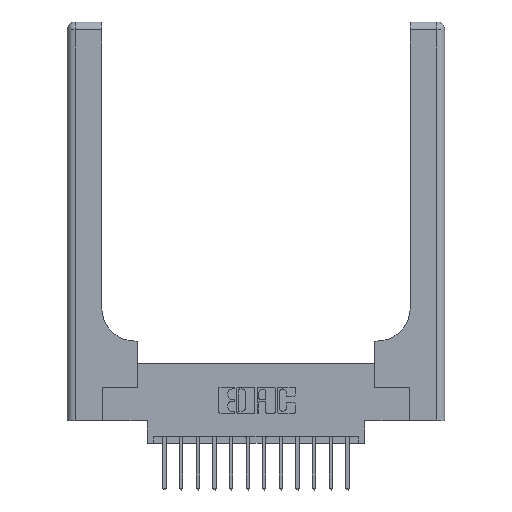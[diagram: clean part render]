
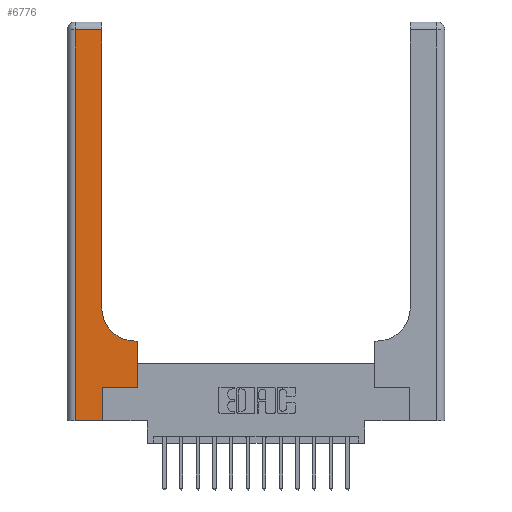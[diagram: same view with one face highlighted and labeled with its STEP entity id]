
A CAD part, top view. The second image highlights one B-rep face of the part: STEP entity #6776.
In plain terms, the highlighted planar face has unit normal (0, 0, 1).
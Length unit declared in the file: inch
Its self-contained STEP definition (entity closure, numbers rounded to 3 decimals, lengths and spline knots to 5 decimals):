
#59 = DIRECTION ( 'NONE',  ( 1., 0., 0. ) ) ;
#504 = DIRECTION ( 'NONE',  ( 0., 1., 0. ) ) ;
#699 = CARTESIAN_POINT ( 'NONE',  ( 0.265, 0.25, 0.37 ) ) ;
#1008 = PLANE ( 'NONE',  #9609 ) ;
#1213 = VERTEX_POINT ( 'NONE', #1940 ) ;
#1661 = EDGE_CURVE ( 'NONE', #13261, #1213, #16543, .T. ) ;
#1783 = LINE ( 'NONE', #15184, #11985 ) ;
#1837 = CARTESIAN_POINT ( 'NONE',  ( 0.06, 3., 0.37 ) ) ;
#1850 = FACE_OUTER_BOUND ( 'NONE', #15285, .T. ) ;
#1940 = CARTESIAN_POINT ( 'NONE',  ( 0.528, 0.25, 0.37 ) ) ;
#2339 = EDGE_CURVE ( 'NONE', #14521, #10930, #16321, .T. ) ;
#2341 = CARTESIAN_POINT ( 'NONE',  ( 0.26, 0.6, 0.37 ) ) ;
#2517 = CIRCLE ( 'NONE', #5534, 0.25 ) ;
#2592 = CARTESIAN_POINT ( 'NONE',  ( 0.528, 0.25, 0.37 ) ) ;
#2735 = CARTESIAN_POINT ( 'NONE',  ( 0.06, 2.94, 0.37 ) ) ;
#2907 = VECTOR ( 'NONE', #6356, 39.37008 ) ;
#3152 = CARTESIAN_POINT ( 'NONE',  ( 0.265, 0.25, 0.37 ) ) ;
#3167 = ORIENTED_EDGE ( 'NONE', *, *, #15888, .T. ) ;
#3273 = EDGE_CURVE ( 'NONE', #9309, #14521, #8649, .T. ) ;
#3549 = VECTOR ( 'NONE', #15789, 39.37008 ) ;
#3654 = LINE ( 'NONE', #2592, #6794 ) ;
#3976 = LINE ( 'NONE', #9172, #3549 ) ;
#4113 = VERTEX_POINT ( 'NONE', #9343 ) ;
#4684 = VERTEX_POINT ( 'NONE', #16342 ) ;
#4693 = DIRECTION ( 'NONE',  ( 1., 0., 0. ) ) ;
#5178 = ORIENTED_EDGE ( 'NONE', *, *, #13541, .T. ) ;
#5183 = VERTEX_POINT ( 'NONE', #13406 ) ;
#5332 = ORIENTED_EDGE ( 'NONE', *, *, #3273, .T. ) ;
#5534 = AXIS2_PLACEMENT_3D ( 'NONE', #15979, #8024, #59 ) ;
#5975 = ORIENTED_EDGE ( 'NONE', *, *, #2339, .T. ) ;
#6150 = EDGE_CURVE ( 'NONE', #4113, #14596, #3976, .T. ) ;
#6356 = DIRECTION ( 'NONE',  ( -1., 0., 0. ) ) ;
#6461 = LINE ( 'NONE', #2341, #2907 ) ;
#6776 = ADVANCED_FACE ( 'NONE', ( #1850 ), #1008, .F. ) ;
#6794 = VECTOR ( 'NONE', #13196, 39.37008 ) ;
#7263 = ORIENTED_EDGE ( 'NONE', *, *, #9973, .T. ) ;
#7431 = CARTESIAN_POINT ( 'NONE',  ( 0.26, 2.94, 0.37 ) ) ;
#7546 = ORIENTED_EDGE ( 'NONE', *, *, #8370, .T. ) ;
#7697 = DIRECTION ( 'NONE',  ( 0., 0., -1. ) ) ;
#7896 = DIRECTION ( 'NONE',  ( 1., 0., 0. ) ) ;
#8024 = DIRECTION ( 'NONE',  ( 0., 0., -1. ) ) ;
#8370 = EDGE_CURVE ( 'NONE', #10930, #13261, #10602, .T. ) ;
#8649 = LINE ( 'NONE', #1837, #9076 ) ;
#9076 = VECTOR ( 'NONE', #13798, 39.37008 ) ;
#9172 = CARTESIAN_POINT ( 'NONE',  ( 0.26, 3., 0.37 ) ) ;
#9239 = CARTESIAN_POINT ( 'NONE',  ( 0., 0., 0.37 ) ) ;
#9309 = VERTEX_POINT ( 'NONE', #2735 ) ;
#9343 = CARTESIAN_POINT ( 'NONE',  ( 0.26, 0.85, 0.37 ) ) ;
#9609 = AXIS2_PLACEMENT_3D ( 'NONE', #15654, #7697, #16988 ) ;
#9973 = EDGE_CURVE ( 'NONE', #14596, #9309, #1783, .T. ) ;
#10602 = LINE ( 'NONE', #16417, #13731 ) ;
#10930 = VERTEX_POINT ( 'NONE', #14872 ) ;
#11985 = VECTOR ( 'NONE', #16503, 39.37008 ) ;
#12174 = ORIENTED_EDGE ( 'NONE', *, *, #6150, .T. ) ;
#12600 = CARTESIAN_POINT ( 'NONE',  ( 0.06, 0., 0.37 ) ) ;
#12798 = VECTOR ( 'NONE', #7896, 39.37008 ) ;
#13014 = EDGE_CURVE ( 'NONE', #5183, #4113, #2517, .T. ) ;
#13028 = VECTOR ( 'NONE', #4693, 39.37008 ) ;
#13103 = ORIENTED_EDGE ( 'NONE', *, *, #1661, .T. ) ;
#13196 = DIRECTION ( 'NONE',  ( 0., 1., 0. ) ) ;
#13261 = VERTEX_POINT ( 'NONE', #3152 ) ;
#13406 = CARTESIAN_POINT ( 'NONE',  ( 0.51, 0.6, 0.37 ) ) ;
#13541 = EDGE_CURVE ( 'NONE', #4684, #5183, #6461, .T. ) ;
#13731 = VECTOR ( 'NONE', #504, 39.37008 ) ;
#13798 = DIRECTION ( 'NONE',  ( 0., -1., 0. ) ) ;
#14521 = VERTEX_POINT ( 'NONE', #12600 ) ;
#14596 = VERTEX_POINT ( 'NONE', #7431 ) ;
#14872 = CARTESIAN_POINT ( 'NONE',  ( 0.265, 0., 0.37 ) ) ;
#15184 = CARTESIAN_POINT ( 'NONE',  ( 0., 2.94, 0.37 ) ) ;
#15285 = EDGE_LOOP ( 'NONE', ( #12174, #7263, #5332, #5975, #7546, #13103, #3167, #5178, #16004 ) ) ;
#15654 = CARTESIAN_POINT ( 'NONE',  ( 0., 3., 0.37 ) ) ;
#15789 = DIRECTION ( 'NONE',  ( 0., 1., 0. ) ) ;
#15888 = EDGE_CURVE ( 'NONE', #1213, #4684, #3654, .T. ) ;
#15979 = CARTESIAN_POINT ( 'NONE',  ( 0.51, 0.85, 0.37 ) ) ;
#16004 = ORIENTED_EDGE ( 'NONE', *, *, #13014, .T. ) ;
#16321 = LINE ( 'NONE', #9239, #12798 ) ;
#16342 = CARTESIAN_POINT ( 'NONE',  ( 0.528, 0.6, 0.37 ) ) ;
#16417 = CARTESIAN_POINT ( 'NONE',  ( 0.265, 0., 0.37 ) ) ;
#16503 = DIRECTION ( 'NONE',  ( -1., 0., 0. ) ) ;
#16543 = LINE ( 'NONE', #699, #13028 ) ;
#16988 = DIRECTION ( 'NONE',  ( -1., 0., 0. ) ) ;
